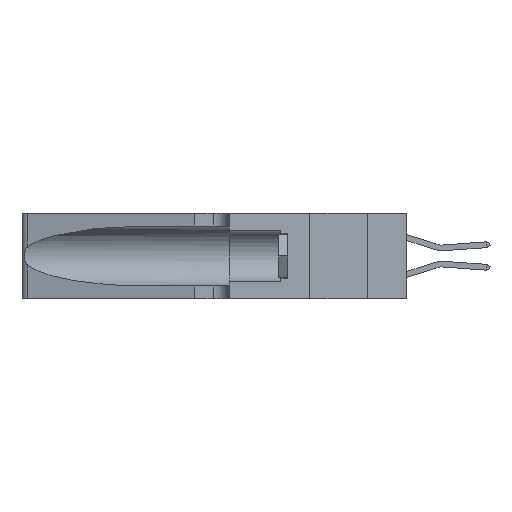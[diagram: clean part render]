
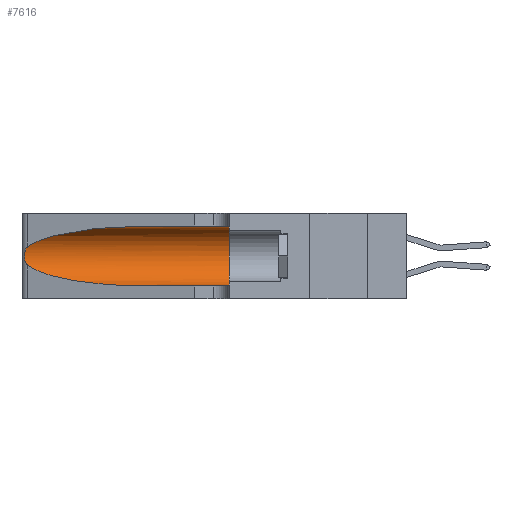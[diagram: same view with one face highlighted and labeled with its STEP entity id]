
A CAD part, left-side view. The second image highlights one B-rep face of the part: STEP entity #7616.
In plain terms, the highlighted cylindrical face has radius 3.308 mm (diameter 6.617 mm), a partial arc.
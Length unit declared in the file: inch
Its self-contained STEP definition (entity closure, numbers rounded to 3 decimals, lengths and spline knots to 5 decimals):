
#100 = AXIS2_PLACEMENT_3D ( 'NONE', #17133, #38675, #20251 ) ;
#553 = AXIS2_PLACEMENT_3D ( 'NONE', #29198, #1428, #7594 ) ;
#1012 = VERTEX_POINT ( 'NONE', #2959 ) ;
#1428 = DIRECTION ( 'NONE',  ( 0., -1., 0. ) ) ;
#1827 = EDGE_CURVE ( 'NONE', #3519, #31316, #23059, .T. ) ;
#2133 = CARTESIAN_POINT ( 'NONE',  ( 0.1305, 1.61858, 0.31525 ) ) ;
#2878 = CARTESIAN_POINT ( 'NONE',  ( 0.26017, 1.23833, 0.17102 ) ) ;
#2959 = CARTESIAN_POINT ( 'NONE',  ( 0.1305, 0.35, 0.31525 ) ) ;
#3017 = CARTESIAN_POINT ( 'NONE',  ( 0.2373, 1.15595, 0.08982 ) ) ;
#3078 = ORIENTED_EDGE ( 'NONE', *, *, #36887, .T. ) ;
#3519 = VERTEX_POINT ( 'NONE', #30875 ) ;
#3801 =( BOUNDED_CURVE ( )  B_SPLINE_CURVE ( 3, ( #6223, #3017, #12438, #34013 ),
 .UNSPECIFIED., .F., .F. ) 
 B_SPLINE_CURVE_WITH_KNOTS ( ( 4, 4 ),
 ( 3.44316, 4.71239 ),
 .UNSPECIFIED. ) 
 CURVE ( )  GEOMETRIC_REPRESENTATION_ITEM ( )  RATIONAL_B_SPLINE_CURVE ( ( 1., 0.87, 0.87, 1. ) ) 
 REPRESENTATION_ITEM ( '' )  );
#5830 = CARTESIAN_POINT ( 'NONE',  ( 0.25639, 1.23184, 0.21858 ) ) ;
#5954 = CARTESIAN_POINT ( 'NONE',  ( 0.25789, 1.23486, 0.15765 ) ) ;
#5980 = CYLINDRICAL_SURFACE ( 'NONE', #553, 0.13025 ) ;
#6223 = CARTESIAN_POINT ( 'NONE',  ( 0.25487, 1.22718, 0.14631 ) ) ;
#6757 = B_SPLINE_CURVE_WITH_KNOTS ( 'NONE', 3,
 ( #33625, #30532, #5830, #15139, #36718, #18274, #39792, #21379, #2878, #24465, #5954, #27579, #9080, #30662 ),
 .UNSPECIFIED., .F., .F.,
 ( 4, 2, 2, 2, 2, 2, 4 ),
 ( 0., 0.00027, 0.00053, 0.00107, 0.0016, 0.00187, 0.00214 ),
 .UNSPECIFIED. ) ;
#7594 = DIRECTION ( 'NONE',  ( 0., 0., -1. ) ) ;
#7616 = ADVANCED_FACE ( 'NONE', ( #23409 ), #5980, .F. ) ;
#8354 = CIRCLE ( 'NONE', #100, 0.13025 ) ;
#8398 = VECTOR ( 'NONE', #14404, 39.37008 ) ;
#9080 = CARTESIAN_POINT ( 'NONE',  ( 0.25555, 1.22993, 0.14849 ) ) ;
#11828 = EDGE_LOOP ( 'NONE', ( #14408, #36381, #3078, #37748, #35227, #24399 ) ) ;
#12074 = CARTESIAN_POINT ( 'NONE',  ( 0.2373, 1.15595, 0.28018 ) ) ;
#12438 = CARTESIAN_POINT ( 'NONE',  ( 0.18966, 0.96281, 0.05475 ) ) ;
#13017 = CARTESIAN_POINT ( 'NONE',  ( 0.1305, 1.61858, 0.05475 ) ) ;
#13151 = EDGE_CURVE ( 'NONE', #32131, #25258, #6757, .T. ) ;
#14287 = EDGE_CURVE ( 'NONE', #26509, #1012, #24821, .T. ) ;
#14404 = DIRECTION ( 'NONE',  ( 0., -1., 0. ) ) ;
#14408 = ORIENTED_EDGE ( 'NONE', *, *, #26704, .T. ) ;
#15139 = CARTESIAN_POINT ( 'NONE',  ( 0.25787, 1.23484, 0.2124 ) ) ;
#17133 = CARTESIAN_POINT ( 'NONE',  ( 0.1305, 0.35, 0.185 ) ) ;
#18274 = CARTESIAN_POINT ( 'NONE',  ( 0.26018, 1.23835, 0.19895 ) ) ;
#20060 = CARTESIAN_POINT ( 'NONE',  ( 0.25487, 1.22718, 0.14631 ) ) ;
#20251 = DIRECTION ( 'NONE',  ( 0., 0., 1. ) ) ;
#20871 = CARTESIAN_POINT ( 'NONE',  ( 0.25487, 1.22718, 0.22369 ) ) ;
#21379 = CARTESIAN_POINT ( 'NONE',  ( 0.26075, 1.23896, 0.178 ) ) ;
#23059 = LINE ( 'NONE', #13017, #24014 ) ;
#23074 = CARTESIAN_POINT ( 'NONE',  ( 0.1305, 0.35, 0.05475 ) ) ;
#23409 = FACE_OUTER_BOUND ( 'NONE', #11828, .T. ) ;
#24014 = VECTOR ( 'NONE', #34584, 39.37008 ) ;
#24399 = ORIENTED_EDGE ( 'NONE', *, *, #14287, .F. ) ;
#24465 = CARTESIAN_POINT ( 'NONE',  ( 0.25856, 1.23593, 0.16098 ) ) ;
#24821 = LINE ( 'NONE', #2133, #8398 ) ;
#25258 = VERTEX_POINT ( 'NONE', #20060 ) ;
#25354 =( BOUNDED_CURVE ( )  B_SPLINE_CURVE ( 3, ( #35839, #27483, #12074, #33666 ),
 .UNSPECIFIED., .F., .T. ) 
 B_SPLINE_CURVE_WITH_KNOTS ( ( 4, 4 ),
 ( 1.5708, 2.84003 ),
 .UNSPECIFIED. ) 
 CURVE ( )  GEOMETRIC_REPRESENTATION_ITEM ( )  RATIONAL_B_SPLINE_CURVE ( ( 1., 0.87, 0.87, 1. ) ) 
 REPRESENTATION_ITEM ( '' )  );
#25761 = CARTESIAN_POINT ( 'NONE',  ( 0.1305, 0.72297, 0.31525 ) ) ;
#26509 = VERTEX_POINT ( 'NONE', #25761 ) ;
#26704 = EDGE_CURVE ( 'NONE', #26509, #32131, #25354, .T. ) ;
#27483 = CARTESIAN_POINT ( 'NONE',  ( 0.18966, 0.96281, 0.31525 ) ) ;
#27579 = CARTESIAN_POINT ( 'NONE',  ( 0.25639, 1.23186, 0.15144 ) ) ;
#29198 = CARTESIAN_POINT ( 'NONE',  ( 0.1305, 1.61858, 0.185 ) ) ;
#30532 = CARTESIAN_POINT ( 'NONE',  ( 0.25555, 1.22994, 0.2215 ) ) ;
#30662 = CARTESIAN_POINT ( 'NONE',  ( 0.25487, 1.22718, 0.14631 ) ) ;
#30875 = CARTESIAN_POINT ( 'NONE',  ( 0.1305, 0.72297, 0.05475 ) ) ;
#31316 = VERTEX_POINT ( 'NONE', #23074 ) ;
#31354 = EDGE_CURVE ( 'NONE', #1012, #31316, #8354, .T. ) ;
#32131 = VERTEX_POINT ( 'NONE', #20871 ) ;
#33625 = CARTESIAN_POINT ( 'NONE',  ( 0.25487, 1.22718, 0.22369 ) ) ;
#33666 = CARTESIAN_POINT ( 'NONE',  ( 0.25487, 1.22718, 0.22369 ) ) ;
#34013 = CARTESIAN_POINT ( 'NONE',  ( 0.1305, 0.72297, 0.05475 ) ) ;
#34584 = DIRECTION ( 'NONE',  ( 0., -1., 0. ) ) ;
#35227 = ORIENTED_EDGE ( 'NONE', *, *, #31354, .F. ) ;
#35839 = CARTESIAN_POINT ( 'NONE',  ( 0.1305, 0.72297, 0.31525 ) ) ;
#36381 = ORIENTED_EDGE ( 'NONE', *, *, #13151, .T. ) ;
#36718 = CARTESIAN_POINT ( 'NONE',  ( 0.25854, 1.2359, 0.20912 ) ) ;
#36887 = EDGE_CURVE ( 'NONE', #25258, #3519, #3801, .T. ) ;
#37748 = ORIENTED_EDGE ( 'NONE', *, *, #1827, .T. ) ;
#38675 = DIRECTION ( 'NONE',  ( 0., 1., 0. ) ) ;
#39792 = CARTESIAN_POINT ( 'NONE',  ( 0.26075, 1.23896, 0.19203 ) ) ;
